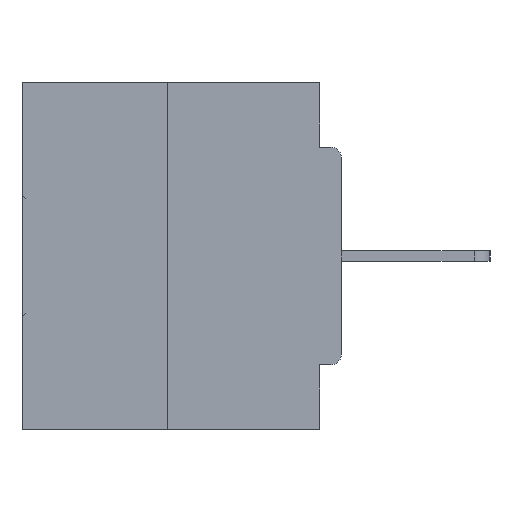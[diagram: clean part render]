
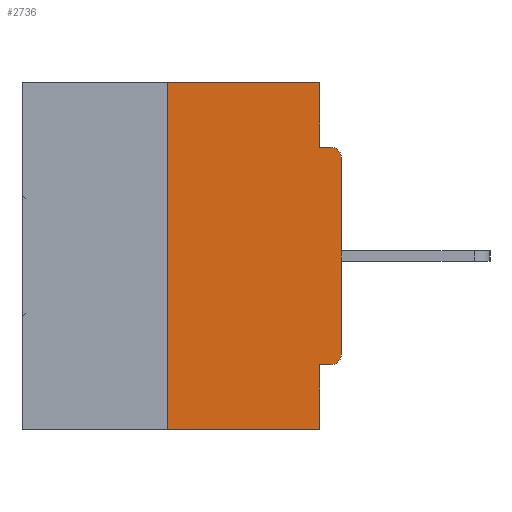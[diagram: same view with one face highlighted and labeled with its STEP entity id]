
A CAD part, left-side view. The second image highlights one B-rep face of the part: STEP entity #2736.
In plain terms, the highlighted planar face has unit normal (-1, 0, 0).
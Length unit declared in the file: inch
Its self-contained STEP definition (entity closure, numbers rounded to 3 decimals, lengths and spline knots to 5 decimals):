
#170 = VERTEX_POINT ( 'NONE', #36152 ) ;
#738 = AXIS2_PLACEMENT_3D ( 'NONE', #7536, #27915, #10436 ) ;
#975 = VECTOR ( 'NONE', #2981, 39.37008 ) ;
#1164 = DIRECTION ( 'NONE',  ( 0., -1., 0. ) ) ;
#1486 = EDGE_CURVE ( 'NONE', #1985, #25359, #36301, .T. ) ;
#1985 = VERTEX_POINT ( 'NONE', #32901 ) ;
#2223 = CIRCLE ( 'NONE', #738, 0.015 ) ;
#2325 = VERTEX_POINT ( 'NONE', #18228 ) ;
#2713 = EDGE_CURVE ( 'NONE', #25633, #18213, #8836, .T. ) ;
#2736 = ADVANCED_FACE ( 'NONE', ( #32111 ), #23546, .F. ) ;
#2981 = DIRECTION ( 'NONE',  ( 0., -1., 0. ) ) ;
#4071 = EDGE_CURVE ( 'NONE', #2325, #7049, #22469, .T. ) ;
#4405 = VERTEX_POINT ( 'NONE', #30824 ) ;
#4494 = LINE ( 'NONE', #12300, #34626 ) ;
#4515 = ORIENTED_EDGE ( 'NONE', *, *, #1486, .T. ) ;
#4808 = VERTEX_POINT ( 'NONE', #26954 ) ;
#4974 = VECTOR ( 'NONE', #16909, 39.37008 ) ;
#5507 = ORIENTED_EDGE ( 'NONE', *, *, #9239, .F. ) ;
#5705 = AXIS2_PLACEMENT_3D ( 'NONE', #17702, #6096, #26457 ) ;
#5924 = LINE ( 'NONE', #31578, #4974 ) ;
#6031 = VECTOR ( 'NONE', #1164, 39.37008 ) ;
#6096 = DIRECTION ( 'NONE',  ( 1., 0., 0. ) ) ;
#6445 = VECTOR ( 'NONE', #11286, 39.37008 ) ;
#6935 = VECTOR ( 'NONE', #23216, 39.37008 ) ;
#7049 = VERTEX_POINT ( 'NONE', #29250 ) ;
#7423 = LINE ( 'NONE', #24287, #22046 ) ;
#7536 = CARTESIAN_POINT ( 'NONE',  ( 0., 0.015, -0.1085 ) ) ;
#8836 = LINE ( 'NONE', #29164, #975 ) ;
#9239 = EDGE_CURVE ( 'NONE', #32736, #2325, #20687, .T. ) ;
#9668 = CARTESIAN_POINT ( 'NONE',  ( 0., 0., -0.3915 ) ) ;
#9917 = ORIENTED_EDGE ( 'NONE', *, *, #16505, .F. ) ;
#10436 = DIRECTION ( 'NONE',  ( 0., 0., -1. ) ) ;
#11219 = ORIENTED_EDGE ( 'NONE', *, *, #2713, .T. ) ;
#11228 = EDGE_CURVE ( 'NONE', #25633, #32736, #5924, .T. ) ;
#11286 = DIRECTION ( 'NONE',  ( 0., 0., -1. ) ) ;
#11487 = EDGE_CURVE ( 'NONE', #1985, #170, #4494, .T. ) ;
#12300 = CARTESIAN_POINT ( 'NONE',  ( 0., 0., -0.4065 ) ) ;
#16505 = EDGE_CURVE ( 'NONE', #170, #18213, #28769, .T. ) ;
#16909 = DIRECTION ( 'NONE',  ( 0., 0., 1. ) ) ;
#17568 = EDGE_CURVE ( 'NONE', #4405, #4808, #2223, .T. ) ;
#17702 = CARTESIAN_POINT ( 'NONE',  ( 0., 0.46, 0. ) ) ;
#18213 = VERTEX_POINT ( 'NONE', #36662 ) ;
#18228 = CARTESIAN_POINT ( 'NONE',  ( 0., 0.031, 0. ) ) ;
#18341 = VECTOR ( 'NONE', #29619, 39.37008 ) ;
#18761 = CARTESIAN_POINT ( 'NONE',  ( 0., 0.46, 0. ) ) ;
#19149 = AXIS2_PLACEMENT_3D ( 'NONE', #29144, #32822, #32774 ) ;
#19779 = CARTESIAN_POINT ( 'NONE',  ( 0., 0.25, -0.5 ) ) ;
#20687 = LINE ( 'NONE', #18761, #6031 ) ;
#22046 = VECTOR ( 'NONE', #27213, 39.37008 ) ;
#22469 = LINE ( 'NONE', #35055, #6935 ) ;
#22801 = EDGE_LOOP ( 'NONE', ( #5507, #30809, #11219, #9917, #29606, #4515, #23000, #33507, #29327, #25026 ) ) ;
#23000 = ORIENTED_EDGE ( 'NONE', *, *, #29064, .T. ) ;
#23216 = DIRECTION ( 'NONE',  ( 0., 0., -1. ) ) ;
#23546 = PLANE ( 'NONE',  #5705 ) ;
#24287 = CARTESIAN_POINT ( 'NONE',  ( 0., 0., 0. ) ) ;
#25026 = ORIENTED_EDGE ( 'NONE', *, *, #4071, .F. ) ;
#25359 = VERTEX_POINT ( 'NONE', #9668 ) ;
#25633 = VERTEX_POINT ( 'NONE', #19779 ) ;
#26457 = DIRECTION ( 'NONE',  ( 0., 0., -1. ) ) ;
#26660 = CARTESIAN_POINT ( 'NONE',  ( 0., 0., -0.0935 ) ) ;
#26954 = CARTESIAN_POINT ( 'NONE',  ( 0., 0.015, -0.0935 ) ) ;
#27213 = DIRECTION ( 'NONE',  ( 0., 0., 1. ) ) ;
#27915 = DIRECTION ( 'NONE',  ( -1., 0., 0. ) ) ;
#28768 = CARTESIAN_POINT ( 'NONE',  ( 0., 0.031, -0.5 ) ) ;
#28769 = LINE ( 'NONE', #28768, #6445 ) ;
#29064 = EDGE_CURVE ( 'NONE', #25359, #4405, #7423, .T. ) ;
#29144 = CARTESIAN_POINT ( 'NONE',  ( 0., 0.015, -0.3915 ) ) ;
#29164 = CARTESIAN_POINT ( 'NONE',  ( 0., 0.46, -0.5 ) ) ;
#29250 = CARTESIAN_POINT ( 'NONE',  ( 0., 0.031, -0.0935 ) ) ;
#29327 = ORIENTED_EDGE ( 'NONE', *, *, #29575, .F. ) ;
#29575 = EDGE_CURVE ( 'NONE', #7049, #4808, #33837, .T. ) ;
#29606 = ORIENTED_EDGE ( 'NONE', *, *, #11487, .F. ) ;
#29619 = DIRECTION ( 'NONE',  ( 0., -1., 0. ) ) ;
#30809 = ORIENTED_EDGE ( 'NONE', *, *, #11228, .F. ) ;
#30824 = CARTESIAN_POINT ( 'NONE',  ( 0., 0., -0.1085 ) ) ;
#31578 = CARTESIAN_POINT ( 'NONE',  ( 0., 0.25, 0. ) ) ;
#32111 = FACE_OUTER_BOUND ( 'NONE', #22801, .T. ) ;
#32732 = DIRECTION ( 'NONE',  ( 0., 1., 0. ) ) ;
#32736 = VERTEX_POINT ( 'NONE', #33619 ) ;
#32774 = DIRECTION ( 'NONE',  ( 0., 0., -1. ) ) ;
#32822 = DIRECTION ( 'NONE',  ( -1., 0., 0. ) ) ;
#32901 = CARTESIAN_POINT ( 'NONE',  ( 0., 0.015, -0.4065 ) ) ;
#33507 = ORIENTED_EDGE ( 'NONE', *, *, #17568, .T. ) ;
#33619 = CARTESIAN_POINT ( 'NONE',  ( 0., 0.25, 0. ) ) ;
#33837 = LINE ( 'NONE', #26660, #18341 ) ;
#34626 = VECTOR ( 'NONE', #32732, 39.37008 ) ;
#35055 = CARTESIAN_POINT ( 'NONE',  ( 0., 0.031, 0. ) ) ;
#36152 = CARTESIAN_POINT ( 'NONE',  ( 0., 0.031, -0.4065 ) ) ;
#36301 = CIRCLE ( 'NONE', #19149, 0.015 ) ;
#36662 = CARTESIAN_POINT ( 'NONE',  ( 0., 0.031, -0.5 ) ) ;
